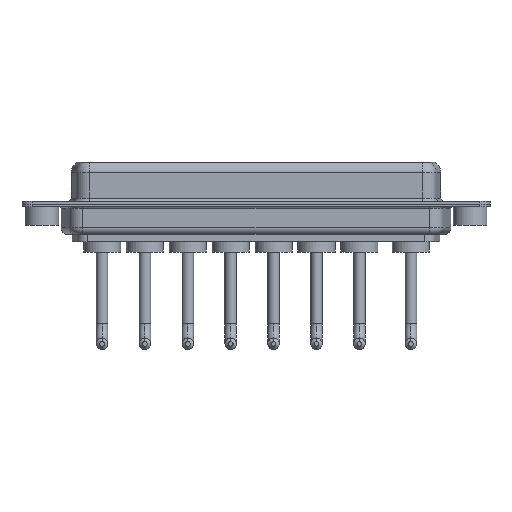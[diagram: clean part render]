
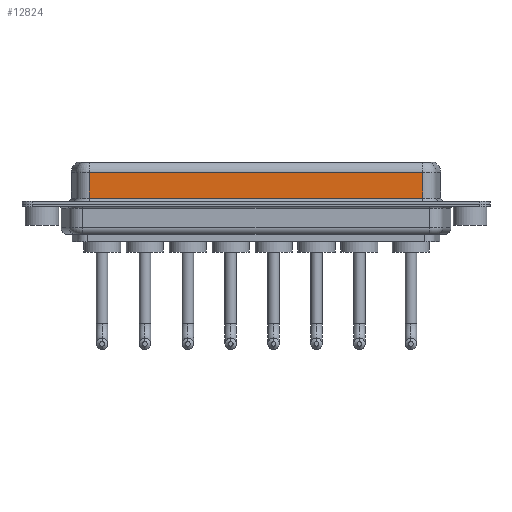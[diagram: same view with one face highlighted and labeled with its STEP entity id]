
A CAD part, front view. The second image highlights one B-rep face of the part: STEP entity #12824.
In plain terms, the highlighted planar face has unit normal (0, -1, 0).
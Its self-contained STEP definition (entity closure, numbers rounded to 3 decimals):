
#1012 = CARTESIAN_POINT ( 'NONE',  ( 7.038, -3.95, 6.4 ) ) ;
#1479 = VERTEX_POINT ( 'NONE', #6589 ) ;
#2431 = LINE ( 'NONE', #7393, #6870 ) ;
#2750 = VERTEX_POINT ( 'NONE', #10416 ) ;
#2760 = CARTESIAN_POINT ( 'NONE',  ( 56.462, -3.95, 6.4 ) ) ;
#2885 = FACE_OUTER_BOUND ( 'NONE', #9170, .T. ) ;
#2985 = DIRECTION ( 'NONE',  ( 0., 0., -1. ) ) ;
#3329 = LINE ( 'NONE', #5342, #4677 ) ;
#3511 = CARTESIAN_POINT ( 'NONE',  ( 56.462, -3.95, 4.65 ) ) ;
#4151 = DIRECTION ( 'NONE',  ( -1., 0., 0. ) ) ;
#4316 = DIRECTION ( 'NONE',  ( 0., 0., -1. ) ) ;
#4628 = PLANE ( 'NONE',  #6551 ) ;
#4677 = VECTOR ( 'NONE', #4151, 1000. ) ;
#4694 = DIRECTION ( 'NONE',  ( 0., 0., 1. ) ) ;
#4755 = ORIENTED_EDGE ( 'NONE', *, *, #8161, .T. ) ;
#5084 = EDGE_CURVE ( 'NONE', #1479, #12830, #8163, .T. ) ;
#5342 = CARTESIAN_POINT ( 'NONE',  ( 56.462, -3.95, 4.65 ) ) ;
#5703 = VECTOR ( 'NONE', #8207, 1000. ) ;
#5711 = CARTESIAN_POINT ( 'NONE',  ( 7.038, -3.95, 0.9 ) ) ;
#6551 = AXIS2_PLACEMENT_3D ( 'NONE', #2760, #7727, #4694 ) ;
#6589 = CARTESIAN_POINT ( 'NONE',  ( 7.038, -3.95, 4.65 ) ) ;
#6648 = ORIENTED_EDGE ( 'NONE', *, *, #8650, .F. ) ;
#6737 = VERTEX_POINT ( 'NONE', #3511 ) ;
#6870 = VECTOR ( 'NONE', #4316, 1000. ) ;
#7393 = CARTESIAN_POINT ( 'NONE',  ( 56.462, -3.95, 6.4 ) ) ;
#7727 = DIRECTION ( 'NONE',  ( 0., 1., 0. ) ) ;
#8161 = EDGE_CURVE ( 'NONE', #6737, #1479, #3329, .T. ) ;
#8163 = LINE ( 'NONE', #1012, #8411 ) ;
#8207 = DIRECTION ( 'NONE',  ( 1., 0., 0. ) ) ;
#8288 = ORIENTED_EDGE ( 'NONE', *, *, #12583, .T. ) ;
#8411 = VECTOR ( 'NONE', #2985, 1000. ) ;
#8650 = EDGE_CURVE ( 'NONE', #6737, #2750, #2431, .T. ) ;
#9170 = EDGE_LOOP ( 'NONE', ( #6648, #4755, #13173, #8288 ) ) ;
#10233 = CARTESIAN_POINT ( 'NONE',  ( 56.462, -3.95, 0.9 ) ) ;
#10416 = CARTESIAN_POINT ( 'NONE',  ( 56.462, -3.95, 0.9 ) ) ;
#12583 = EDGE_CURVE ( 'NONE', #12830, #2750, #13319, .T. ) ;
#12824 = ADVANCED_FACE ( 'NONE', ( #2885 ), #4628, .F. ) ;
#12830 = VERTEX_POINT ( 'NONE', #5711 ) ;
#13173 = ORIENTED_EDGE ( 'NONE', *, *, #5084, .T. ) ;
#13319 = LINE ( 'NONE', #10233, #5703 ) ;
